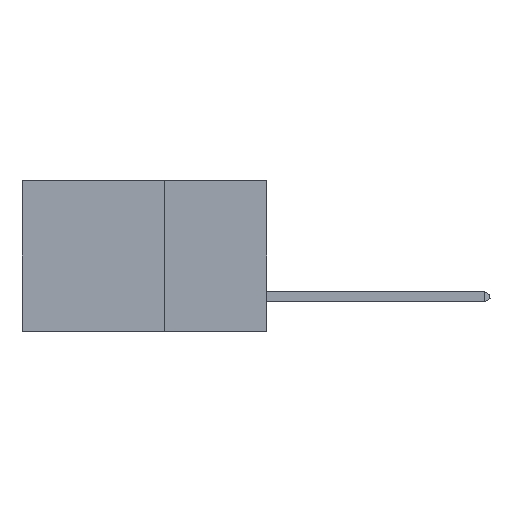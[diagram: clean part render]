
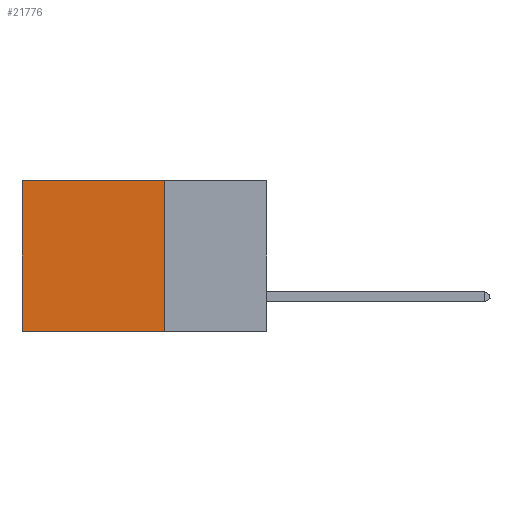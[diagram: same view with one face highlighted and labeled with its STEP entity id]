
A CAD part, left-side view. The second image highlights one B-rep face of the part: STEP entity #21776.
In plain terms, the highlighted planar face has unit normal (-1, 0, 0).
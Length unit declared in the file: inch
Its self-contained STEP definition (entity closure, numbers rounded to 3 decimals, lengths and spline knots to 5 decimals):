
#91 = CARTESIAN_POINT ( 'NONE',  ( 0.2875, 0.25, 0. ) ) ;
#229 = VERTEX_POINT ( 'NONE', #4699 ) ;
#814 = EDGE_CURVE ( 'NONE', #10689, #13064, #5276, .T. ) ;
#1405 = AXIS2_PLACEMENT_3D ( 'NONE', #16608, #4809, #24461 ) ;
#2846 = ORIENTED_EDGE ( 'NONE', *, *, #814, .T. ) ;
#4699 = CARTESIAN_POINT ( 'NONE',  ( 0.2875, 0.25, -0.37 ) ) ;
#4809 = DIRECTION ( 'NONE',  ( 1., 0., 0. ) ) ;
#5112 = LINE ( 'NONE', #91, #23531 ) ;
#5276 = LINE ( 'NONE', #19503, #10501 ) ;
#5956 = CARTESIAN_POINT ( 'NONE',  ( 0.2875, 0.6, 0. ) ) ;
#6099 = EDGE_CURVE ( 'NONE', #10689, #229, #5112, .T. ) ;
#6286 = VECTOR ( 'NONE', #9997, 39.37008 ) ;
#6934 = EDGE_CURVE ( 'NONE', #229, #10382, #10584, .T. ) ;
#7096 = FACE_OUTER_BOUND ( 'NONE', #8850, .T. ) ;
#7436 = DIRECTION ( 'NONE',  ( 0., 1., 0. ) ) ;
#7840 = VECTOR ( 'NONE', #7436, 39.37008 ) ;
#8850 = EDGE_LOOP ( 'NONE', ( #17748, #15647, #9896, #2846 ) ) ;
#9896 = ORIENTED_EDGE ( 'NONE', *, *, #6099, .F. ) ;
#9997 = DIRECTION ( 'NONE',  ( 0., 0., -1. ) ) ;
#10290 = LINE ( 'NONE', #5956, #6286 ) ;
#10382 = VERTEX_POINT ( 'NONE', #18376 ) ;
#10501 = VECTOR ( 'NONE', #12327, 39.37008 ) ;
#10584 = LINE ( 'NONE', #19143, #7840 ) ;
#10689 = VERTEX_POINT ( 'NONE', #24778 ) ;
#12327 = DIRECTION ( 'NONE',  ( 0., 1., 0. ) ) ;
#13064 = VERTEX_POINT ( 'NONE', #21039 ) ;
#15647 = ORIENTED_EDGE ( 'NONE', *, *, #6934, .F. ) ;
#16608 = CARTESIAN_POINT ( 'NONE',  ( 0.2875, 0.25, 0. ) ) ;
#17748 = ORIENTED_EDGE ( 'NONE', *, *, #19346, .T. ) ;
#17825 = DIRECTION ( 'NONE',  ( 0., 0., -1. ) ) ;
#18376 = CARTESIAN_POINT ( 'NONE',  ( 0.2875, 0.6, -0.37 ) ) ;
#19143 = CARTESIAN_POINT ( 'NONE',  ( 0.2875, 0.25, -0.37 ) ) ;
#19346 = EDGE_CURVE ( 'NONE', #13064, #10382, #10290, .T. ) ;
#19503 = CARTESIAN_POINT ( 'NONE',  ( 0.2875, 0.25, 0. ) ) ;
#21039 = CARTESIAN_POINT ( 'NONE',  ( 0.2875, 0.6, 0. ) ) ;
#21776 = ADVANCED_FACE ( 'NONE', ( #7096 ), #22397, .F. ) ;
#22397 = PLANE ( 'NONE',  #1405 ) ;
#23531 = VECTOR ( 'NONE', #17825, 39.37008 ) ;
#24461 = DIRECTION ( 'NONE',  ( 0., 0., -1. ) ) ;
#24778 = CARTESIAN_POINT ( 'NONE',  ( 0.2875, 0.25, 0. ) ) ;
